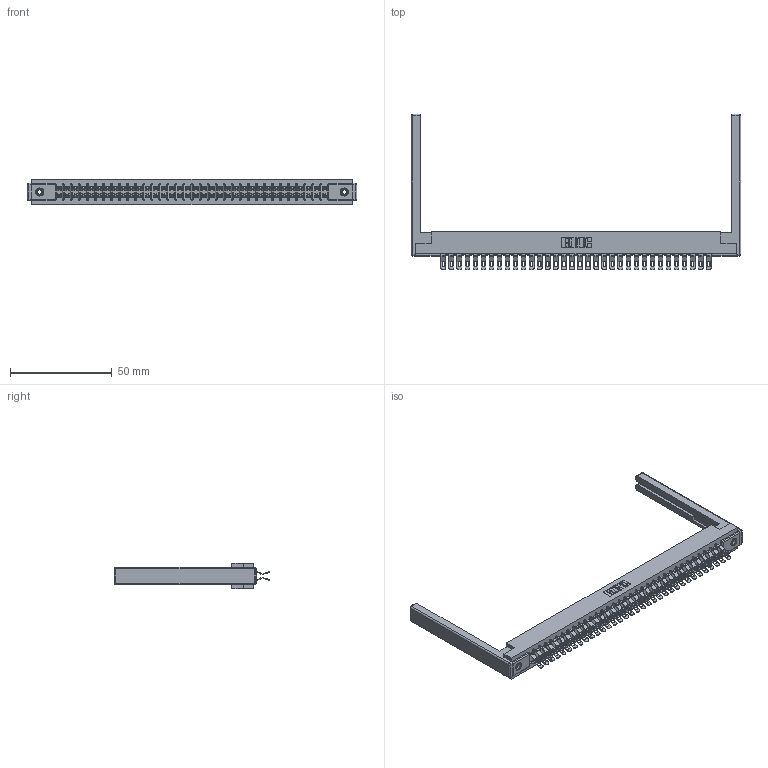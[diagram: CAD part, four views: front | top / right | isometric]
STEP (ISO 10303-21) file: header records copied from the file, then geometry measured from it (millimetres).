
FILE_DESCRIPTION (( 'STEP AP203' ), '1' );
FILE_NAME ('357-068-555-268.STEP', '2019-09-19T09:42:13', ( '' ), ( '' ), 'SwSTEP 2.0', 'SolidWorks 2016', '' );
FILE_SCHEMA (( 'CONFIG_CONTROL_DESIGN' ));
Length unit declared in the file: inch
Products named in the file (5): 357-068-555-268; 307-290-001_555; 345-250-001_345-250-001-102; 307-220-068; 307 Part_.156 Dia Mounting Holes
Assembly tree (73 placements, depth 2):
  357-068-555-268
    307 Part_.156 Dia Mounting Holes
    307-290-001_555  x68
    307-220-068  x2
    345-250-001_345-250-001-102  x2
Bounding box: 162.15 x 76.71 x 12.7 mm (x, y, z)
Volume: 21769.6 mm3; surface area: 26221.4 mm2
Topology: 73 solids, 73 shells, 4455 faces, 13021 edges, 8474 vertices
Faces by surface type: plane 2470, cylinder 1891, sphere 78, cone 12, torus 4
Entity records: 34518 total; most frequent: CARTESIAN_POINT 5631, ORIENTED_EDGE 5574, DIRECTION 5541, EDGE_CURVE 2787, VECTOR 2121, LINE 2121, VERTEX_POINT 1800, AXIS2_PLACEMENT_3D 1710
